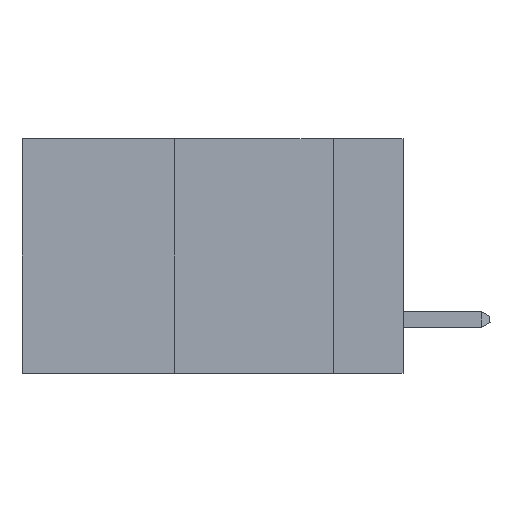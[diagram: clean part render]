
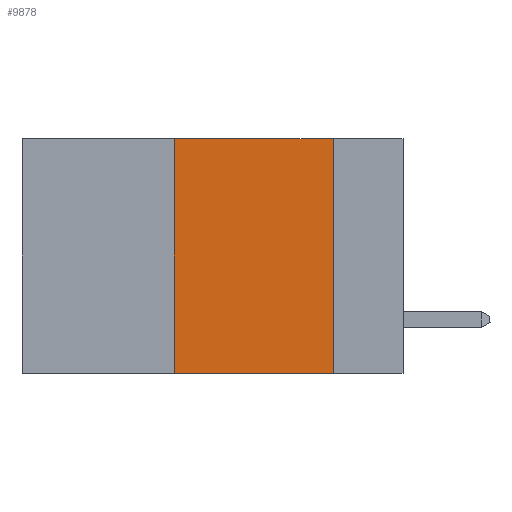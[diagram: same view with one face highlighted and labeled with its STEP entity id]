
A CAD part, left-side view. The second image highlights one B-rep face of the part: STEP entity #9878.
In plain terms, the highlighted planar face has unit normal (-1, 0, 0).
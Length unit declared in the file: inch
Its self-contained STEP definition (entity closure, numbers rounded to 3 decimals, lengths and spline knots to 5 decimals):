
#428 = LINE ( 'NONE', #7838, #10309 ) ;
#478 = VECTOR ( 'NONE', #1207, 39.37008 ) ;
#808 = EDGE_CURVE ( 'NONE', #1210, #9716, #3215, .T. ) ;
#1128 = EDGE_CURVE ( 'NONE', #6027, #1210, #5623, .T. ) ;
#1207 = DIRECTION ( 'NONE',  ( 0., 0., 1. ) ) ;
#1210 = VERTEX_POINT ( 'NONE', #9682 ) ;
#1216 = PLANE ( 'NONE',  #12264 ) ;
#1538 = LINE ( 'NONE', #7844, #8968 ) ;
#1804 = EDGE_CURVE ( 'NONE', #6027, #7000, #1538, .T. ) ;
#1981 = CARTESIAN_POINT ( 'NONE',  ( 0., 0.11, 0. ) ) ;
#2477 = VECTOR ( 'NONE', #2636, 39.37008 ) ;
#2636 = DIRECTION ( 'NONE',  ( 0., -1., 0. ) ) ;
#3047 = DIRECTION ( 'NONE',  ( 0., -1., 0. ) ) ;
#3215 = LINE ( 'NONE', #6473, #2477 ) ;
#4039 = DIRECTION ( 'NONE',  ( 1., 0., 0. ) ) ;
#5623 = LINE ( 'NONE', #7948, #478 ) ;
#6027 = VERTEX_POINT ( 'NONE', #6594 ) ;
#6473 = CARTESIAN_POINT ( 'NONE',  ( 0., 0.6, 0. ) ) ;
#6594 = CARTESIAN_POINT ( 'NONE',  ( 0., 0.36, -0.37 ) ) ;
#7000 = VERTEX_POINT ( 'NONE', #11423 ) ;
#7177 = ORIENTED_EDGE ( 'NONE', *, *, #1804, .T. ) ;
#7700 = ORIENTED_EDGE ( 'NONE', *, *, #7983, .F. ) ;
#7838 = CARTESIAN_POINT ( 'NONE',  ( 0., 0.11, 0. ) ) ;
#7844 = CARTESIAN_POINT ( 'NONE',  ( 0., 0.6, -0.37 ) ) ;
#7948 = CARTESIAN_POINT ( 'NONE',  ( 0., 0.36, 0. ) ) ;
#7956 = CARTESIAN_POINT ( 'NONE',  ( 0., 0.6, 0. ) ) ;
#7983 = EDGE_CURVE ( 'NONE', #9716, #7000, #428, .T. ) ;
#8334 = ORIENTED_EDGE ( 'NONE', *, *, #1128, .F. ) ;
#8885 = ORIENTED_EDGE ( 'NONE', *, *, #808, .F. ) ;
#8968 = VECTOR ( 'NONE', #3047, 39.37008 ) ;
#9437 = FACE_OUTER_BOUND ( 'NONE', #10795, .T. ) ;
#9682 = CARTESIAN_POINT ( 'NONE',  ( 0., 0.36, 0. ) ) ;
#9716 = VERTEX_POINT ( 'NONE', #1981 ) ;
#9878 = ADVANCED_FACE ( 'NONE', ( #9437 ), #1216, .F. ) ;
#10309 = VECTOR ( 'NONE', #11752, 39.37008 ) ;
#10795 = EDGE_LOOP ( 'NONE', ( #7700, #8885, #8334, #7177 ) ) ;
#10855 = DIRECTION ( 'NONE',  ( 0., 0., -1. ) ) ;
#11423 = CARTESIAN_POINT ( 'NONE',  ( 0., 0.11, -0.37 ) ) ;
#11752 = DIRECTION ( 'NONE',  ( 0., 0., -1. ) ) ;
#12264 = AXIS2_PLACEMENT_3D ( 'NONE', #7956, #4039, #10855 ) ;
